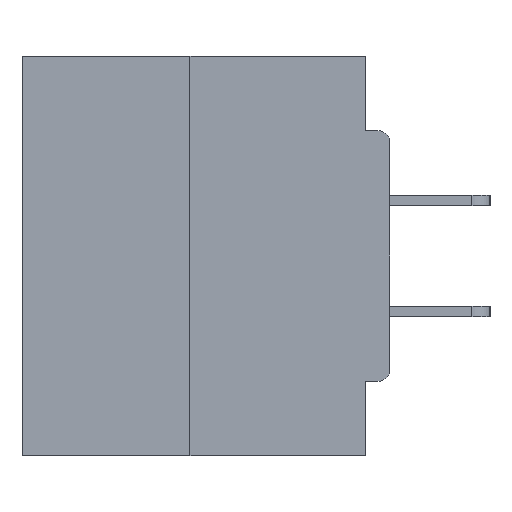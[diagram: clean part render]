
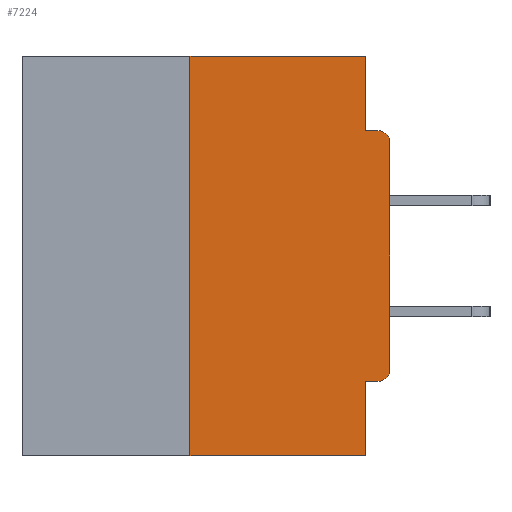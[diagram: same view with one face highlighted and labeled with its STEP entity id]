
A CAD part, left-side view. The second image highlights one B-rep face of the part: STEP entity #7224.
In plain terms, the highlighted planar face has unit normal (-1, 0, 0).
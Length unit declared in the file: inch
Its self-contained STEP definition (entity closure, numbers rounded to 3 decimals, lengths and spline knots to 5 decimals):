
#224 = LINE ( 'NONE', #6415, #19508 ) ;
#505 = DIRECTION ( 'NONE',  ( 0., 0., 1. ) ) ;
#1331 = EDGE_CURVE ( 'NONE', #27806, #35338, #23754, .T. ) ;
#1446 = VERTEX_POINT ( 'NONE', #18662 ) ;
#2145 = DIRECTION ( 'NONE',  ( 0., 0., -1. ) ) ;
#3577 = ORIENTED_EDGE ( 'NONE', *, *, #9398, .T. ) ;
#3582 = CARTESIAN_POINT ( 'NONE',  ( 0., 0., -0.4065 ) ) ;
#4701 = VERTEX_POINT ( 'NONE', #20773 ) ;
#5007 = CARTESIAN_POINT ( 'NONE',  ( 0., 0.015, -0.4065 ) ) ;
#5638 = DIRECTION ( 'NONE',  ( 0., -1., 0. ) ) ;
#6415 = CARTESIAN_POINT ( 'NONE',  ( 0., 0.46, -0.5 ) ) ;
#6777 = DIRECTION ( 'NONE',  ( 0., 1., 0. ) ) ;
#7224 = ADVANCED_FACE ( 'NONE', ( #33720 ), #35971, .F. ) ;
#7435 = VECTOR ( 'NONE', #5638, 39.37008 ) ;
#7580 = DIRECTION ( 'NONE',  ( 0., -1., 0. ) ) ;
#7854 = DIRECTION ( 'NONE',  ( -1., 0., 0. ) ) ;
#7946 = LINE ( 'NONE', #19416, #24747 ) ;
#9246 = EDGE_CURVE ( 'NONE', #4701, #1446, #32495, .T. ) ;
#9375 = ORIENTED_EDGE ( 'NONE', *, *, #21063, .F. ) ;
#9398 = EDGE_CURVE ( 'NONE', #25514, #18896, #11759, .T. ) ;
#9401 = DIRECTION ( 'NONE',  ( -1., 0., 0. ) ) ;
#9622 = CARTESIAN_POINT ( 'NONE',  ( 0., 0.25, 0. ) ) ;
#9854 = VECTOR ( 'NONE', #505, 39.37008 ) ;
#9875 = VECTOR ( 'NONE', #21122, 39.37008 ) ;
#11713 = CARTESIAN_POINT ( 'NONE',  ( 0., 0.031, 0. ) ) ;
#11759 = LINE ( 'NONE', #31354, #9854 ) ;
#11997 = ORIENTED_EDGE ( 'NONE', *, *, #23529, .T. ) ;
#12108 = CARTESIAN_POINT ( 'NONE',  ( 0., 0., -0.3915 ) ) ;
#12129 = CARTESIAN_POINT ( 'NONE',  ( 0., 0., -0.1085 ) ) ;
#12910 = DIRECTION ( 'NONE',  ( 0., 0., -1. ) ) ;
#13219 = CARTESIAN_POINT ( 'NONE',  ( 0., 0.46, 0. ) ) ;
#15191 = CARTESIAN_POINT ( 'NONE',  ( 0., 0.031, -0.5 ) ) ;
#15875 = ORIENTED_EDGE ( 'NONE', *, *, #9246, .F. ) ;
#15986 = EDGE_CURVE ( 'NONE', #18896, #21561, #20482, .T. ) ;
#17576 = VECTOR ( 'NONE', #12910, 39.37008 ) ;
#17647 = LINE ( 'NONE', #29134, #7435 ) ;
#18034 = CARTESIAN_POINT ( 'NONE',  ( 0., 0.031, 0. ) ) ;
#18281 = EDGE_CURVE ( 'NONE', #31961, #21561, #7946, .T. ) ;
#18662 = CARTESIAN_POINT ( 'NONE',  ( 0., 0.031, -0.5 ) ) ;
#18813 = ORIENTED_EDGE ( 'NONE', *, *, #36473, .T. ) ;
#18896 = VERTEX_POINT ( 'NONE', #12129 ) ;
#19416 = CARTESIAN_POINT ( 'NONE',  ( 0., 0., -0.0935 ) ) ;
#19508 = VECTOR ( 'NONE', #20519, 39.37008 ) ;
#19664 = ORIENTED_EDGE ( 'NONE', *, *, #15986, .T. ) ;
#20482 = CIRCLE ( 'NONE', #34879, 0.015 ) ;
#20519 = DIRECTION ( 'NONE',  ( 0., -1., 0. ) ) ;
#20526 = CARTESIAN_POINT ( 'NONE',  ( 0., 0.015, -0.3915 ) ) ;
#20557 = AXIS2_PLACEMENT_3D ( 'NONE', #20526, #9401, #34805 ) ;
#20663 = VECTOR ( 'NONE', #32757, 39.37008 ) ;
#20773 = CARTESIAN_POINT ( 'NONE',  ( 0., 0.031, -0.4065 ) ) ;
#21063 = EDGE_CURVE ( 'NONE', #28501, #31961, #21281, .T. ) ;
#21122 = DIRECTION ( 'NONE',  ( 0., 0., 1. ) ) ;
#21143 = EDGE_CURVE ( 'NONE', #21690, #4701, #23901, .T. ) ;
#21260 = ORIENTED_EDGE ( 'NONE', *, *, #22684, .F. ) ;
#21281 = LINE ( 'NONE', #18034, #20663 ) ;
#21561 = VERTEX_POINT ( 'NONE', #30573 ) ;
#21690 = VERTEX_POINT ( 'NONE', #5007 ) ;
#22088 = DIRECTION ( 'NONE',  ( 1., 0., 0. ) ) ;
#22684 = EDGE_CURVE ( 'NONE', #35338, #28501, #17647, .T. ) ;
#23529 = EDGE_CURVE ( 'NONE', #27806, #1446, #224, .T. ) ;
#23746 = EDGE_LOOP ( 'NONE', ( #21260, #28240, #11997, #15875, #23941, #18813, #3577, #19664, #28102, #9375 ) ) ;
#23754 = LINE ( 'NONE', #9622, #9875 ) ;
#23901 = LINE ( 'NONE', #3582, #25484 ) ;
#23941 = ORIENTED_EDGE ( 'NONE', *, *, #21143, .F. ) ;
#24747 = VECTOR ( 'NONE', #7580, 39.37008 ) ;
#25484 = VECTOR ( 'NONE', #6777, 39.37008 ) ;
#25514 = VERTEX_POINT ( 'NONE', #12108 ) ;
#25970 = CIRCLE ( 'NONE', #20557, 0.015 ) ;
#27617 = DIRECTION ( 'NONE',  ( 0., 0., -1. ) ) ;
#27806 = VERTEX_POINT ( 'NONE', #27855 ) ;
#27855 = CARTESIAN_POINT ( 'NONE',  ( 0., 0.25, -0.5 ) ) ;
#28102 = ORIENTED_EDGE ( 'NONE', *, *, #18281, .F. ) ;
#28240 = ORIENTED_EDGE ( 'NONE', *, *, #1331, .F. ) ;
#28501 = VERTEX_POINT ( 'NONE', #11713 ) ;
#29134 = CARTESIAN_POINT ( 'NONE',  ( 0., 0.46, 0. ) ) ;
#30573 = CARTESIAN_POINT ( 'NONE',  ( 0., 0.015, -0.0935 ) ) ;
#31354 = CARTESIAN_POINT ( 'NONE',  ( 0., 0., 0. ) ) ;
#31961 = VERTEX_POINT ( 'NONE', #35514 ) ;
#32495 = LINE ( 'NONE', #15191, #17576 ) ;
#32757 = DIRECTION ( 'NONE',  ( 0., 0., -1. ) ) ;
#33046 = AXIS2_PLACEMENT_3D ( 'NONE', #13219, #22088, #2145 ) ;
#33626 = CARTESIAN_POINT ( 'NONE',  ( 0., 0.015, -0.1085 ) ) ;
#33720 = FACE_OUTER_BOUND ( 'NONE', #23746, .T. ) ;
#34805 = DIRECTION ( 'NONE',  ( 0., 0., -1. ) ) ;
#34879 = AXIS2_PLACEMENT_3D ( 'NONE', #33626, #7854, #27617 ) ;
#35338 = VERTEX_POINT ( 'NONE', #36336 ) ;
#35514 = CARTESIAN_POINT ( 'NONE',  ( 0., 0.031, -0.0935 ) ) ;
#35971 = PLANE ( 'NONE',  #33046 ) ;
#36336 = CARTESIAN_POINT ( 'NONE',  ( 0., 0.25, 0. ) ) ;
#36473 = EDGE_CURVE ( 'NONE', #21690, #25514, #25970, .T. ) ;
